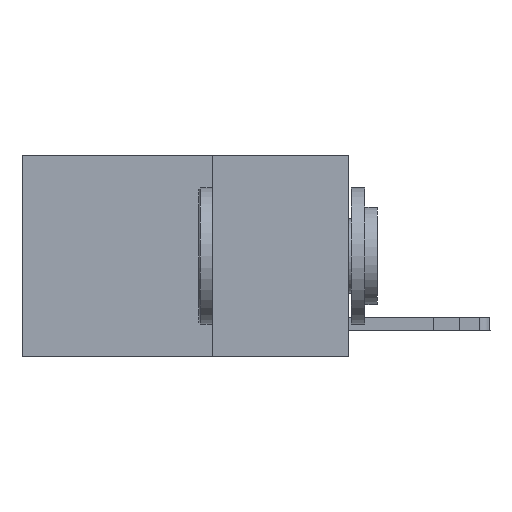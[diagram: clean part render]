
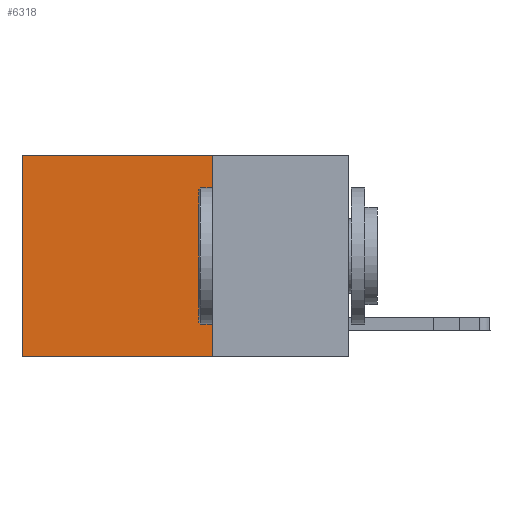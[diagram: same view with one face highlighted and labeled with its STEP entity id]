
A CAD part, left-side view. The second image highlights one B-rep face of the part: STEP entity #6318.
In plain terms, the highlighted planar face has unit normal (-1, 0, 0).
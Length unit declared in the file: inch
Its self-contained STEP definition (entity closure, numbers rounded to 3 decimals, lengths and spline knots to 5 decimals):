
#462 = CARTESIAN_POINT ( 'NONE',  ( 0.2625, 0.25, -0.37 ) ) ;
#515 = VERTEX_POINT ( 'NONE', #13319 ) ;
#2953 = FACE_OUTER_BOUND ( 'NONE', #6732, .T. ) ;
#3067 = EDGE_CURVE ( 'NONE', #515, #12367, #15136, .T. ) ;
#4314 = DIRECTION ( 'NONE',  ( 0., 0., -1. ) ) ;
#4596 = ORIENTED_EDGE ( 'NONE', *, *, #13395, .T. ) ;
#4611 = DIRECTION ( 'NONE',  ( 0., 0., -1. ) ) ;
#4721 = LINE ( 'NONE', #4941, #19134 ) ;
#4941 = CARTESIAN_POINT ( 'NONE',  ( 0.2625, 0.6, 0. ) ) ;
#6318 = ADVANCED_FACE ( 'NONE', ( #2953 ), #9914, .F. ) ;
#6732 = EDGE_LOOP ( 'NONE', ( #4596, #11422, #8913, #9444 ) ) ;
#7579 = AXIS2_PLACEMENT_3D ( 'NONE', #9805, #8122, #4314 ) ;
#8122 = DIRECTION ( 'NONE',  ( 1., 0., 0. ) ) ;
#8196 = CARTESIAN_POINT ( 'NONE',  ( 0.2625, 0.6, 0. ) ) ;
#8279 = DIRECTION ( 'NONE',  ( 0., 1., 0. ) ) ;
#8676 = CARTESIAN_POINT ( 'NONE',  ( 0.2625, 0.25, 0. ) ) ;
#8913 = ORIENTED_EDGE ( 'NONE', *, *, #16134, .F. ) ;
#9111 = VERTEX_POINT ( 'NONE', #19232 ) ;
#9444 = ORIENTED_EDGE ( 'NONE', *, *, #3067, .T. ) ;
#9805 = CARTESIAN_POINT ( 'NONE',  ( 0.2625, 0.25, 0. ) ) ;
#9914 = PLANE ( 'NONE',  #7579 ) ;
#11422 = ORIENTED_EDGE ( 'NONE', *, *, #13189, .F. ) ;
#12367 = VERTEX_POINT ( 'NONE', #8196 ) ;
#12470 = DIRECTION ( 'NONE',  ( 0., 1., 0. ) ) ;
#13189 = EDGE_CURVE ( 'NONE', #9111, #22027, #15875, .T. ) ;
#13319 = CARTESIAN_POINT ( 'NONE',  ( 0.2625, 0.25, 0. ) ) ;
#13395 = EDGE_CURVE ( 'NONE', #12367, #22027, #4721, .T. ) ;
#13662 = CARTESIAN_POINT ( 'NONE',  ( 0.2625, 0.25, 0. ) ) ;
#15136 = LINE ( 'NONE', #13662, #17570 ) ;
#15241 = VECTOR ( 'NONE', #15535, 39.37008 ) ;
#15535 = DIRECTION ( 'NONE',  ( 0., 0., -1. ) ) ;
#15875 = LINE ( 'NONE', #462, #20932 ) ;
#16134 = EDGE_CURVE ( 'NONE', #515, #9111, #20500, .T. ) ;
#17570 = VECTOR ( 'NONE', #8279, 39.37008 ) ;
#19134 = VECTOR ( 'NONE', #4611, 39.37008 ) ;
#19232 = CARTESIAN_POINT ( 'NONE',  ( 0.2625, 0.25, -0.37 ) ) ;
#20500 = LINE ( 'NONE', #8676, #15241 ) ;
#20932 = VECTOR ( 'NONE', #12470, 39.37008 ) ;
#21960 = CARTESIAN_POINT ( 'NONE',  ( 0.2625, 0.6, -0.37 ) ) ;
#22027 = VERTEX_POINT ( 'NONE', #21960 ) ;
